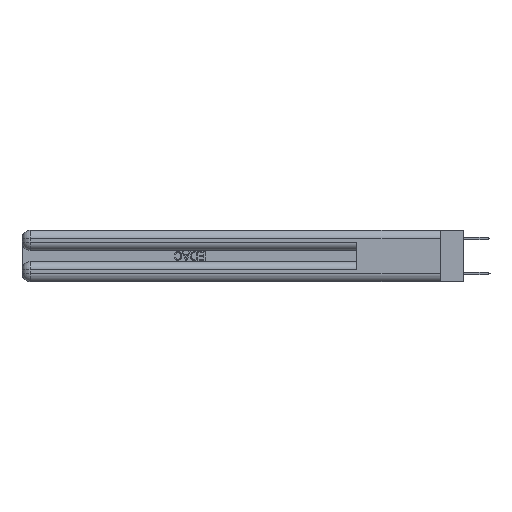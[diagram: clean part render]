
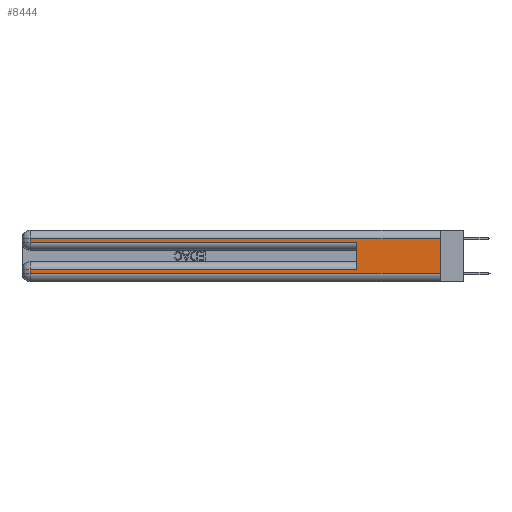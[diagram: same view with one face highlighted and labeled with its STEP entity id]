
A CAD part, left-side view. The second image highlights one B-rep face of the part: STEP entity #8444.
In plain terms, the highlighted planar face has unit normal (-1, 0, 0).
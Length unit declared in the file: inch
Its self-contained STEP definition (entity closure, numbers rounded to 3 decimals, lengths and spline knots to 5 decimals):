
#9 = VERTEX_POINT ( 'NONE', #15711 ) ;
#1248 = VECTOR ( 'NONE', #4467, 39.37008 ) ;
#1532 = LINE ( 'NONE', #19565, #18036 ) ;
#1732 = EDGE_LOOP ( 'NONE', ( #24808, #22466, #18693, #3191, #6873, #26512, #10965, #7612 ) ) ;
#1845 = EDGE_CURVE ( 'NONE', #8733, #11144, #4995, .T. ) ;
#2122 = VERTEX_POINT ( 'NONE', #20164 ) ;
#2304 = CARTESIAN_POINT ( 'NONE',  ( 0., 0., 0.285 ) ) ;
#2606 = CARTESIAN_POINT ( 'NONE',  ( 0., 2.94, 0.06 ) ) ;
#3191 = ORIENTED_EDGE ( 'NONE', *, *, #3705, .T. ) ;
#3343 = EDGE_CURVE ( 'NONE', #24652, #6866, #21647, .T. ) ;
#3705 = EDGE_CURVE ( 'NONE', #2122, #11144, #18429, .T. ) ;
#4467 = DIRECTION ( 'NONE',  ( 0., -1., 0. ) ) ;
#4765 = VERTEX_POINT ( 'NONE', #25226 ) ;
#4995 = LINE ( 'NONE', #27666, #26998 ) ;
#5647 = CARTESIAN_POINT ( 'NONE',  ( 0., 0., 0.06 ) ) ;
#5706 = CARTESIAN_POINT ( 'NONE',  ( 0., 0., 0.31 ) ) ;
#6230 = AXIS2_PLACEMENT_3D ( 'NONE', #25475, #21339, #8600 ) ;
#6399 = PLANE ( 'NONE',  #6230 ) ;
#6447 = LINE ( 'NONE', #23684, #23448 ) ;
#6866 = VERTEX_POINT ( 'NONE', #2606 ) ;
#6873 = ORIENTED_EDGE ( 'NONE', *, *, #1845, .F. ) ;
#7250 = CARTESIAN_POINT ( 'NONE',  ( 0., 0.6, 0.085 ) ) ;
#7612 = ORIENTED_EDGE ( 'NONE', *, *, #15960, .T. ) ;
#8444 = ADVANCED_FACE ( 'NONE', ( #27438 ), #6399, .F. ) ;
#8600 = DIRECTION ( 'NONE',  ( 0., 0., -1. ) ) ;
#8733 = VERTEX_POINT ( 'NONE', #7250 ) ;
#8843 = DIRECTION ( 'NONE',  ( 0., 1., 0. ) ) ;
#9130 = EDGE_CURVE ( 'NONE', #8733, #24652, #6447, .T. ) ;
#10965 = ORIENTED_EDGE ( 'NONE', *, *, #3343, .T. ) ;
#11144 = VERTEX_POINT ( 'NONE', #22217 ) ;
#11967 = VERTEX_POINT ( 'NONE', #14574 ) ;
#13122 = CARTESIAN_POINT ( 'NONE',  ( 0., 2.94, 0.085 ) ) ;
#13184 = DIRECTION ( 'NONE',  ( 0., 0., -1. ) ) ;
#13533 = CARTESIAN_POINT ( 'NONE',  ( 0., 0., 0.37 ) ) ;
#13619 = VECTOR ( 'NONE', #22654, 39.37008 ) ;
#13846 = LINE ( 'NONE', #13533, #16545 ) ;
#14574 = CARTESIAN_POINT ( 'NONE',  ( 0., 2.94, 0.31 ) ) ;
#14774 = EDGE_CURVE ( 'NONE', #4765, #11967, #18959, .T. ) ;
#15711 = CARTESIAN_POINT ( 'NONE',  ( 0., 0., 0.06 ) ) ;
#15960 = EDGE_CURVE ( 'NONE', #6866, #9, #18558, .T. ) ;
#16545 = VECTOR ( 'NONE', #17777, 39.37008 ) ;
#17777 = DIRECTION ( 'NONE',  ( 0., 0., -1. ) ) ;
#18036 = VECTOR ( 'NONE', #13184, 39.37008 ) ;
#18297 = DIRECTION ( 'NONE',  ( 0., 0., -1. ) ) ;
#18429 = LINE ( 'NONE', #2304, #1248 ) ;
#18558 = LINE ( 'NONE', #5647, #13619 ) ;
#18693 = ORIENTED_EDGE ( 'NONE', *, *, #25288, .T. ) ;
#18959 = LINE ( 'NONE', #5706, #24554 ) ;
#19565 = CARTESIAN_POINT ( 'NONE',  ( 0., 2.94, 0.37 ) ) ;
#20164 = CARTESIAN_POINT ( 'NONE',  ( 0., 2.94, 0.285 ) ) ;
#20406 = CARTESIAN_POINT ( 'NONE',  ( 0., 2.94, 0.37 ) ) ;
#20675 = DIRECTION ( 'NONE',  ( 0., 1., 0. ) ) ;
#20995 = VECTOR ( 'NONE', #18297, 39.37008 ) ;
#21339 = DIRECTION ( 'NONE',  ( 1., 0., 0. ) ) ;
#21647 = LINE ( 'NONE', #20406, #20995 ) ;
#22217 = CARTESIAN_POINT ( 'NONE',  ( 0., 0.6, 0.285 ) ) ;
#22466 = ORIENTED_EDGE ( 'NONE', *, *, #14774, .T. ) ;
#22473 = EDGE_CURVE ( 'NONE', #4765, #9, #13846, .T. ) ;
#22654 = DIRECTION ( 'NONE',  ( 0., -1., 0. ) ) ;
#23448 = VECTOR ( 'NONE', #8843, 39.37008 ) ;
#23684 = CARTESIAN_POINT ( 'NONE',  ( 0., 0., 0.085 ) ) ;
#24554 = VECTOR ( 'NONE', #20675, 39.37008 ) ;
#24652 = VERTEX_POINT ( 'NONE', #13122 ) ;
#24808 = ORIENTED_EDGE ( 'NONE', *, *, #22473, .F. ) ;
#25226 = CARTESIAN_POINT ( 'NONE',  ( 0., 0., 0.31 ) ) ;
#25288 = EDGE_CURVE ( 'NONE', #11967, #2122, #1532, .T. ) ;
#25475 = CARTESIAN_POINT ( 'NONE',  ( 0., 0., 0.37 ) ) ;
#26512 = ORIENTED_EDGE ( 'NONE', *, *, #9130, .T. ) ;
#26998 = VECTOR ( 'NONE', #27414, 39.37008 ) ;
#27414 = DIRECTION ( 'NONE',  ( 0., 0., 1. ) ) ;
#27438 = FACE_OUTER_BOUND ( 'NONE', #1732, .T. ) ;
#27666 = CARTESIAN_POINT ( 'NONE',  ( 0., 0.6, 0.145 ) ) ;
